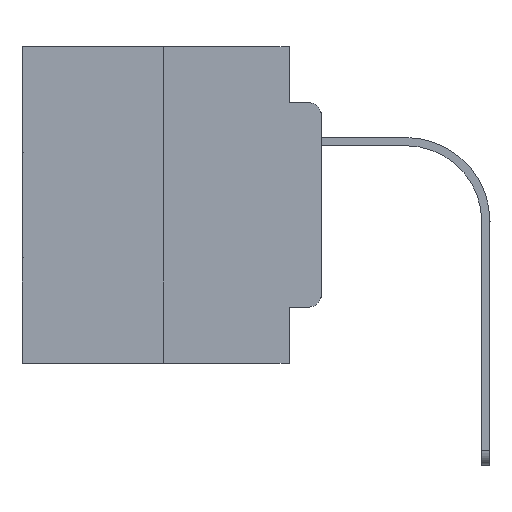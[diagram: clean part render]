
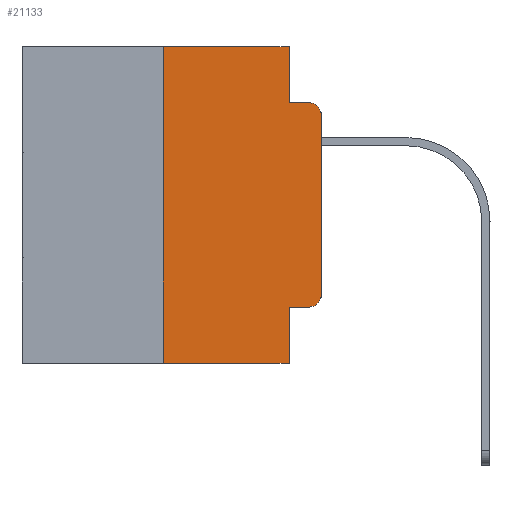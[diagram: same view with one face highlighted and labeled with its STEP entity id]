
A CAD part, left-side view. The second image highlights one B-rep face of the part: STEP entity #21133.
In plain terms, the highlighted planar face has unit normal (-1, 0, 0).
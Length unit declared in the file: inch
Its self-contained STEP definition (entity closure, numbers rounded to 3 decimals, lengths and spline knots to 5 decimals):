
#2260 = CARTESIAN_POINT ( 'NONE',  ( 0., 0.051, 0. ) ) ;
#2856 = LINE ( 'NONE', #25052, #15183 ) ;
#2957 = ORIENTED_EDGE ( 'NONE', *, *, #23372, .F. ) ;
#3000 = VERTEX_POINT ( 'NONE', #3664 ) ;
#3089 = CIRCLE ( 'NONE', #18734, 0.02 ) ;
#3371 = ORIENTED_EDGE ( 'NONE', *, *, #18102, .T. ) ;
#3423 = DIRECTION ( 'NONE',  ( 0., 0., -1. ) ) ;
#3594 = EDGE_CURVE ( 'NONE', #25887, #19341, #11665, .T. ) ;
#3658 = VERTEX_POINT ( 'NONE', #23345 ) ;
#3664 = CARTESIAN_POINT ( 'NONE',  ( 0., 0.25, 0. ) ) ;
#3733 = DIRECTION ( 'NONE',  ( 0., 0., -1. ) ) ;
#3918 = VECTOR ( 'NONE', #11194, 39.37008 ) ;
#4176 = LINE ( 'NONE', #19463, #11007 ) ;
#4922 = VERTEX_POINT ( 'NONE', #8958 ) ;
#5359 = VERTEX_POINT ( 'NONE', #5596 ) ;
#5596 = CARTESIAN_POINT ( 'NONE',  ( 0., 0.02, -0.0885 ) ) ;
#5885 = CARTESIAN_POINT ( 'NONE',  ( 0., 0.02, -0.3915 ) ) ;
#6233 = ORIENTED_EDGE ( 'NONE', *, *, #18199, .T. ) ;
#7092 = VERTEX_POINT ( 'NONE', #26137 ) ;
#8350 = CARTESIAN_POINT ( 'NONE',  ( 0., 0.25, 0. ) ) ;
#8460 = DIRECTION ( 'NONE',  ( 1., 0., 0. ) ) ;
#8599 = DIRECTION ( 'NONE',  ( 0., 0., 1. ) ) ;
#8613 = PLANE ( 'NONE',  #16503 ) ;
#8958 = CARTESIAN_POINT ( 'NONE',  ( 0., 0., -0.1085 ) ) ;
#9526 = ORIENTED_EDGE ( 'NONE', *, *, #3594, .F. ) ;
#9697 = VECTOR ( 'NONE', #19243, 39.37008 ) ;
#9868 = CARTESIAN_POINT ( 'NONE',  ( 0., 0.473, 0. ) ) ;
#10359 = CARTESIAN_POINT ( 'NONE',  ( 0., 0.473, 0. ) ) ;
#10609 = CARTESIAN_POINT ( 'NONE',  ( 0., 0., 0. ) ) ;
#10674 = ORIENTED_EDGE ( 'NONE', *, *, #20269, .T. ) ;
#11007 = VECTOR ( 'NONE', #28226, 39.37008 ) ;
#11194 = DIRECTION ( 'NONE',  ( 0., -1., 0. ) ) ;
#11665 = LINE ( 'NONE', #18440, #19950 ) ;
#12175 = LINE ( 'NONE', #9868, #9697 ) ;
#12547 = LINE ( 'NONE', #8350, #25519 ) ;
#13514 = LINE ( 'NONE', #10609, #19577 ) ;
#13702 = DIRECTION ( 'NONE',  ( 0., 0., -1. ) ) ;
#13839 = EDGE_LOOP ( 'NONE', ( #3371, #20392, #2957, #9526, #19144, #14302, #6233, #14931, #10674, #24255 ) ) ;
#14302 = ORIENTED_EDGE ( 'NONE', *, *, #23293, .F. ) ;
#14684 = DIRECTION ( 'NONE',  ( -1., 0., 0. ) ) ;
#14931 = ORIENTED_EDGE ( 'NONE', *, *, #22874, .F. ) ;
#15183 = VECTOR ( 'NONE', #3423, 39.37008 ) ;
#15605 = VERTEX_POINT ( 'NONE', #23515 ) ;
#15965 = DIRECTION ( 'NONE',  ( 0., 0., -1. ) ) ;
#16050 = EDGE_CURVE ( 'NONE', #3658, #23223, #3089, .T. ) ;
#16242 = DIRECTION ( 'NONE',  ( -1., 0., 0. ) ) ;
#16503 = AXIS2_PLACEMENT_3D ( 'NONE', #10359, #8460, #17421 ) ;
#17076 = CIRCLE ( 'NONE', #21649, 0.02 ) ;
#17421 = DIRECTION ( 'NONE',  ( 0., 0., -1. ) ) ;
#18102 = EDGE_CURVE ( 'NONE', #23223, #4922, #13514, .T. ) ;
#18199 = EDGE_CURVE ( 'NONE', #21958, #15605, #21863, .T. ) ;
#18440 = CARTESIAN_POINT ( 'NONE',  ( 0., 0.051, 0. ) ) ;
#18618 = CARTESIAN_POINT ( 'NONE',  ( 0., 0.25, -0.5 ) ) ;
#18734 = AXIS2_PLACEMENT_3D ( 'NONE', #5885, #14684, #3733 ) ;
#19144 = ORIENTED_EDGE ( 'NONE', *, *, #24597, .F. ) ;
#19243 = DIRECTION ( 'NONE',  ( 0., -1., 0. ) ) ;
#19341 = VERTEX_POINT ( 'NONE', #20004 ) ;
#19463 = CARTESIAN_POINT ( 'NONE',  ( 0., 0.051, -0.0885 ) ) ;
#19501 = DIRECTION ( 'NONE',  ( 0., -1., 0. ) ) ;
#19577 = VECTOR ( 'NONE', #8599, 39.37008 ) ;
#19710 = CARTESIAN_POINT ( 'NONE',  ( 0., 0.473, -0.5 ) ) ;
#19950 = VECTOR ( 'NONE', #13702, 39.37008 ) ;
#20004 = CARTESIAN_POINT ( 'NONE',  ( 0., 0.051, -0.0885 ) ) ;
#20269 = EDGE_CURVE ( 'NONE', #7092, #3658, #28124, .T. ) ;
#20392 = ORIENTED_EDGE ( 'NONE', *, *, #24444, .T. ) ;
#21133 = ADVANCED_FACE ( 'NONE', ( #25773 ), #8613, .F. ) ;
#21207 = DIRECTION ( 'NONE',  ( 0., 0., 1. ) ) ;
#21649 = AXIS2_PLACEMENT_3D ( 'NONE', #22440, #16242, #15965 ) ;
#21803 = CARTESIAN_POINT ( 'NONE',  ( 0., 0.051, -0.4115 ) ) ;
#21863 = LINE ( 'NONE', #19710, #3918 ) ;
#21958 = VERTEX_POINT ( 'NONE', #18618 ) ;
#22440 = CARTESIAN_POINT ( 'NONE',  ( 0., 0.02, -0.1085 ) ) ;
#22821 = CARTESIAN_POINT ( 'NONE',  ( 0., 0., -0.3915 ) ) ;
#22874 = EDGE_CURVE ( 'NONE', #7092, #15605, #2856, .T. ) ;
#23223 = VERTEX_POINT ( 'NONE', #22821 ) ;
#23293 = EDGE_CURVE ( 'NONE', #21958, #3000, #12547, .T. ) ;
#23345 = CARTESIAN_POINT ( 'NONE',  ( 0., 0.02, -0.4115 ) ) ;
#23372 = EDGE_CURVE ( 'NONE', #19341, #5359, #4176, .T. ) ;
#23515 = CARTESIAN_POINT ( 'NONE',  ( 0., 0.051, -0.5 ) ) ;
#24255 = ORIENTED_EDGE ( 'NONE', *, *, #16050, .T. ) ;
#24444 = EDGE_CURVE ( 'NONE', #4922, #5359, #17076, .T. ) ;
#24597 = EDGE_CURVE ( 'NONE', #3000, #25887, #12175, .T. ) ;
#25052 = CARTESIAN_POINT ( 'NONE',  ( 0., 0.051, 0. ) ) ;
#25519 = VECTOR ( 'NONE', #21207, 39.37008 ) ;
#25643 = VECTOR ( 'NONE', #19501, 39.37008 ) ;
#25773 = FACE_OUTER_BOUND ( 'NONE', #13839, .T. ) ;
#25887 = VERTEX_POINT ( 'NONE', #2260 ) ;
#26137 = CARTESIAN_POINT ( 'NONE',  ( 0., 0.051, -0.4115 ) ) ;
#28124 = LINE ( 'NONE', #21803, #25643 ) ;
#28226 = DIRECTION ( 'NONE',  ( 0., -1., 0. ) ) ;
